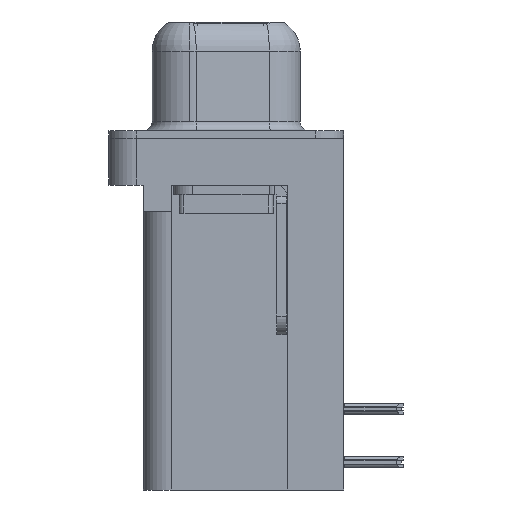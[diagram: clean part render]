
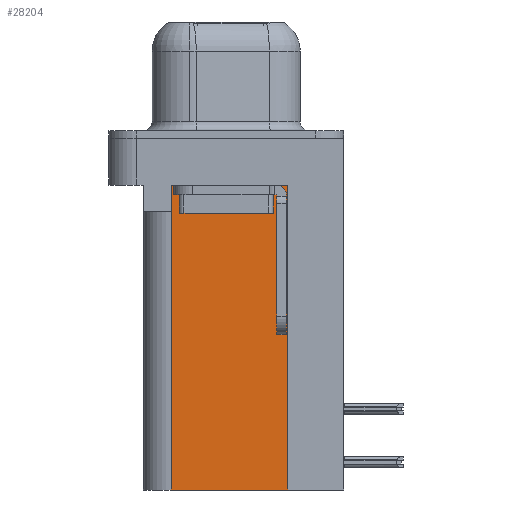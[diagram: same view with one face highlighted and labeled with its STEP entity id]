
A CAD part, left-side view. The second image highlights one B-rep face of the part: STEP entity #28204.
In plain terms, the highlighted planar face has unit normal (-1, 0, 0).
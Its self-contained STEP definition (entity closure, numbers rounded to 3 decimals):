
#717 = FACE_OUTER_BOUND ( 'NONE', #1518, .T. ) ;
#721 = VECTOR ( 'NONE', #20102, 1000. ) ;
#776 = LINE ( 'NONE', #5639, #721 ) ;
#1518 = EDGE_LOOP ( 'NONE', ( #18464, #2622, #26237, #7032, #1709, #10967 ) ) ;
#1709 = ORIENTED_EDGE ( 'NONE', *, *, #16967, .F. ) ;
#2571 = VERTEX_POINT ( 'NONE', #13049 ) ;
#2622 = ORIENTED_EDGE ( 'NONE', *, *, #29981, .T. ) ;
#2791 = DIRECTION ( 'NONE',  ( 0., 0., 1. ) ) ;
#5400 = LINE ( 'NONE', #17225, #22461 ) ;
#5639 = CARTESIAN_POINT ( 'NONE',  ( 3.7, 0., -3.9 ) ) ;
#6009 = VERTEX_POINT ( 'NONE', #9732 ) ;
#6595 = VERTEX_POINT ( 'NONE', #16743 ) ;
#7032 = ORIENTED_EDGE ( 'NONE', *, *, #8415, .F. ) ;
#7064 = AXIS2_PLACEMENT_3D ( 'NONE', #24641, #10200, #26938 ) ;
#7741 = PLANE ( 'NONE',  #7064 ) ;
#8415 = EDGE_CURVE ( 'NONE', #15299, #27062, #20477, .T. ) ;
#9139 = DIRECTION ( 'NONE',  ( 0., 0., 1. ) ) ;
#9510 = DIRECTION ( 'NONE',  ( 0., 1., 0. ) ) ;
#9732 = CARTESIAN_POINT ( 'NONE',  ( 3.7, -3.295, -18.76 ) ) ;
#10200 = DIRECTION ( 'NONE',  ( 1., 0., 0. ) ) ;
#10967 = ORIENTED_EDGE ( 'NONE', *, *, #18174, .T. ) ;
#13049 = CARTESIAN_POINT ( 'NONE',  ( 3.7, 2.895, -2.5 ) ) ;
#14844 = LINE ( 'NONE', #18996, #21179 ) ;
#15299 = VERTEX_POINT ( 'NONE', #16930 ) ;
#16577 = VECTOR ( 'NONE', #26045, 1000. ) ;
#16743 = CARTESIAN_POINT ( 'NONE',  ( 3.7, -3.295, -2.5 ) ) ;
#16930 = CARTESIAN_POINT ( 'NONE',  ( 3.7, 2.925, -18.76 ) ) ;
#16967 = EDGE_CURVE ( 'NONE', #6009, #15299, #21531, .T. ) ;
#17225 = CARTESIAN_POINT ( 'NONE',  ( 3.7, -3.295, -18.76 ) ) ;
#18174 = EDGE_CURVE ( 'NONE', #6009, #6595, #5400, .T. ) ;
#18464 = ORIENTED_EDGE ( 'NONE', *, *, #25708, .T. ) ;
#18620 = CARTESIAN_POINT ( 'NONE',  ( 3.7, 2.925, -18.76 ) ) ;
#18996 = CARTESIAN_POINT ( 'NONE',  ( 3.7, -3.295, -2.5 ) ) ;
#20004 = CARTESIAN_POINT ( 'NONE',  ( 3.7, 2.925, -3.9 ) ) ;
#20102 = DIRECTION ( 'NONE',  ( 0., 1., 0. ) ) ;
#20327 = VECTOR ( 'NONE', #9139, 1000. ) ;
#20477 = LINE ( 'NONE', #18620, #20327 ) ;
#20583 = VERTEX_POINT ( 'NONE', #23504 ) ;
#20705 = CARTESIAN_POINT ( 'NONE',  ( 3.7, 2.895, -3.9 ) ) ;
#21179 = VECTOR ( 'NONE', #9510, 1000. ) ;
#21531 = LINE ( 'NONE', #30600, #16577 ) ;
#21964 = VECTOR ( 'NONE', #25551, 1000. ) ;
#22187 = LINE ( 'NONE', #20705, #21964 ) ;
#22461 = VECTOR ( 'NONE', #2791, 1000. ) ;
#23504 = CARTESIAN_POINT ( 'NONE',  ( 3.7, 2.895, -3.9 ) ) ;
#24641 = CARTESIAN_POINT ( 'NONE',  ( 3.7, -3.295, -18.76 ) ) ;
#25508 = EDGE_CURVE ( 'NONE', #20583, #27062, #776, .T. ) ;
#25551 = DIRECTION ( 'NONE',  ( 0., 0., -1. ) ) ;
#25708 = EDGE_CURVE ( 'NONE', #6595, #2571, #14844, .T. ) ;
#26045 = DIRECTION ( 'NONE',  ( 0., 1., 0. ) ) ;
#26237 = ORIENTED_EDGE ( 'NONE', *, *, #25508, .T. ) ;
#26938 = DIRECTION ( 'NONE',  ( 0., 1., 0. ) ) ;
#27062 = VERTEX_POINT ( 'NONE', #20004 ) ;
#28204 = ADVANCED_FACE ( 'NONE', ( #717 ), #7741, .F. ) ;
#29981 = EDGE_CURVE ( 'NONE', #2571, #20583, #22187, .T. ) ;
#30600 = CARTESIAN_POINT ( 'NONE',  ( 3.7, -3.295, -18.76 ) ) ;
